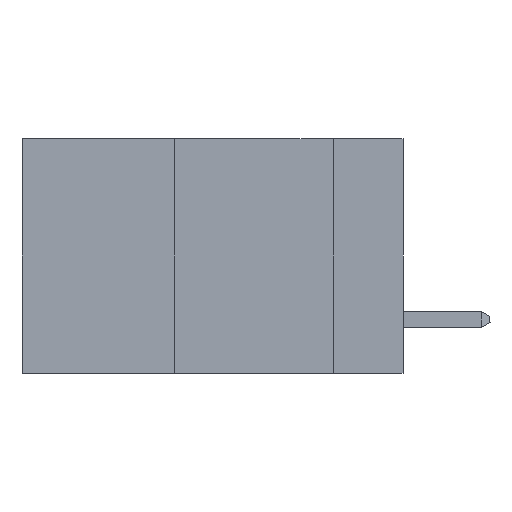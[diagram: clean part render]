
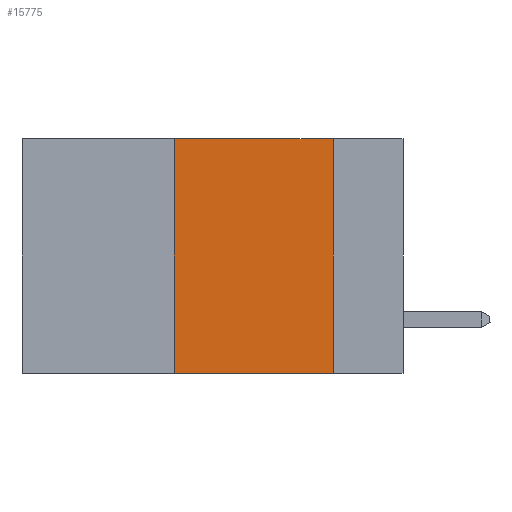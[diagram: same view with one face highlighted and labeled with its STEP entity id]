
A CAD part, left-side view. The second image highlights one B-rep face of the part: STEP entity #15775.
In plain terms, the highlighted planar face has unit normal (-1, 0, 0).
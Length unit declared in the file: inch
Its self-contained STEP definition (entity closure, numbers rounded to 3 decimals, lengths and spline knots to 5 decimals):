
#757 = VERTEX_POINT ( 'NONE', #42246 ) ;
#1409 = EDGE_CURVE ( 'NONE', #35984, #45696, #15869, .T. ) ;
#2148 = CARTESIAN_POINT ( 'NONE',  ( 0., 0.6, 0. ) ) ;
#5501 = CARTESIAN_POINT ( 'NONE',  ( 0., 0.11, -0.37 ) ) ;
#6347 = EDGE_CURVE ( 'NONE', #35984, #757, #7628, .T. ) ;
#7628 = LINE ( 'NONE', #14909, #30366 ) ;
#9203 = ORIENTED_EDGE ( 'NONE', *, *, #12021, .F. ) ;
#10203 = CARTESIAN_POINT ( 'NONE',  ( 0., 0.11, 0. ) ) ;
#11037 = LINE ( 'NONE', #10203, #44314 ) ;
#12021 = EDGE_CURVE ( 'NONE', #757, #21490, #36762, .T. ) ;
#12337 = ORIENTED_EDGE ( 'NONE', *, *, #6347, .F. ) ;
#12675 = CARTESIAN_POINT ( 'NONE',  ( 0., 0.36, -0.37 ) ) ;
#13975 = EDGE_CURVE ( 'NONE', #21490, #45696, #11037, .T. ) ;
#14580 = AXIS2_PLACEMENT_3D ( 'NONE', #30144, #20217, #30748 ) ;
#14909 = CARTESIAN_POINT ( 'NONE',  ( 0., 0.36, 0. ) ) ;
#14995 = DIRECTION ( 'NONE',  ( 0., -1., 0. ) ) ;
#15775 = ADVANCED_FACE ( 'NONE', ( #31419 ), #27202, .F. ) ;
#15869 = LINE ( 'NONE', #29430, #21419 ) ;
#20217 = DIRECTION ( 'NONE',  ( 1., 0., 0. ) ) ;
#21419 = VECTOR ( 'NONE', #14995, 39.37008 ) ;
#21490 = VERTEX_POINT ( 'NONE', #36853 ) ;
#23808 = DIRECTION ( 'NONE',  ( 0., -1., 0. ) ) ;
#27201 = EDGE_LOOP ( 'NONE', ( #34707, #9203, #12337, #42396 ) ) ;
#27202 = PLANE ( 'NONE',  #14580 ) ;
#27858 = DIRECTION ( 'NONE',  ( 0., 0., -1. ) ) ;
#29430 = CARTESIAN_POINT ( 'NONE',  ( 0., 0.6, -0.37 ) ) ;
#30144 = CARTESIAN_POINT ( 'NONE',  ( 0., 0.6, 0. ) ) ;
#30366 = VECTOR ( 'NONE', #32923, 39.37008 ) ;
#30748 = DIRECTION ( 'NONE',  ( 0., 0., -1. ) ) ;
#31419 = FACE_OUTER_BOUND ( 'NONE', #27201, .T. ) ;
#32923 = DIRECTION ( 'NONE',  ( 0., 0., 1. ) ) ;
#34707 = ORIENTED_EDGE ( 'NONE', *, *, #13975, .F. ) ;
#35984 = VERTEX_POINT ( 'NONE', #12675 ) ;
#36762 = LINE ( 'NONE', #2148, #45657 ) ;
#36853 = CARTESIAN_POINT ( 'NONE',  ( 0., 0.11, 0. ) ) ;
#42246 = CARTESIAN_POINT ( 'NONE',  ( 0., 0.36, 0. ) ) ;
#42396 = ORIENTED_EDGE ( 'NONE', *, *, #1409, .T. ) ;
#44314 = VECTOR ( 'NONE', #27858, 39.37008 ) ;
#45657 = VECTOR ( 'NONE', #23808, 39.37008 ) ;
#45696 = VERTEX_POINT ( 'NONE', #5501 ) ;
